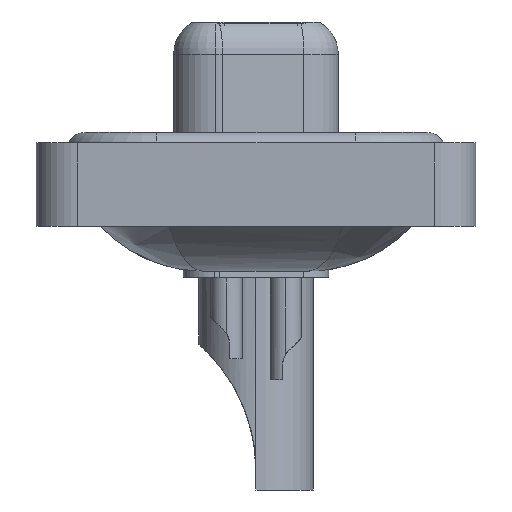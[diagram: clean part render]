
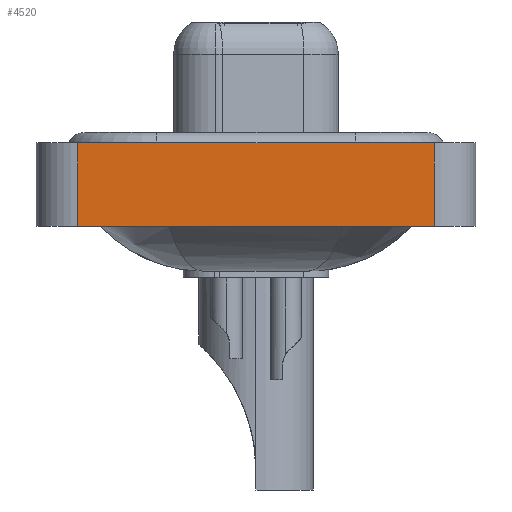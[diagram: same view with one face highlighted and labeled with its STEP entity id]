
A CAD part, left-side view. The second image highlights one B-rep face of the part: STEP entity #4520.
In plain terms, the highlighted planar face has unit normal (-1, 0, 0).
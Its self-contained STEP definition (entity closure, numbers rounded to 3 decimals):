
#196 = VERTEX_POINT ( 'NONE', #629 ) ;
#365 = DIRECTION ( 'NONE',  ( -1., 0., 0. ) ) ;
#629 = CARTESIAN_POINT ( 'NONE',  ( -7.3, -8.55, -3.6 ) ) ;
#1158 = CARTESIAN_POINT ( 'NONE',  ( -7.3, -8.55, -3.6 ) ) ;
#1205 = ORIENTED_EDGE ( 'NONE', *, *, #11827, .T. ) ;
#1836 = DIRECTION ( 'NONE',  ( 0., 0., 1. ) ) ;
#1920 = FACE_OUTER_BOUND ( 'NONE', #9299, .T. ) ;
#3502 = VECTOR ( 'NONE', #10788, 1000. ) ;
#3709 = ORIENTED_EDGE ( 'NONE', *, *, #17572, .F. ) ;
#4520 = ADVANCED_FACE ( 'NONE', ( #1920 ), #15809, .T. ) ;
#4964 = VECTOR ( 'NONE', #1836, 1000. ) ;
#5768 = VERTEX_POINT ( 'NONE', #18923 ) ;
#6378 = CARTESIAN_POINT ( 'NONE',  ( -7.3, -8.55, 0.4 ) ) ;
#6514 = CARTESIAN_POINT ( 'NONE',  ( -7.3, 8.55, 0.4 ) ) ;
#6992 = DIRECTION ( 'NONE',  ( 0., 0., 1. ) ) ;
#8396 = EDGE_CURVE ( 'NONE', #5768, #21709, #9965, .T. ) ;
#9299 = EDGE_LOOP ( 'NONE', ( #16265, #3709, #16435, #1205 ) ) ;
#9965 = LINE ( 'NONE', #22133, #19442 ) ;
#10788 = DIRECTION ( 'NONE',  ( 0., -1., 0. ) ) ;
#11827 = EDGE_CURVE ( 'NONE', #5768, #196, #20378, .T. ) ;
#12151 = CARTESIAN_POINT ( 'NONE',  ( -7.3, -8.55, -3.6 ) ) ;
#12922 = LINE ( 'NONE', #16337, #3502 ) ;
#13296 = DIRECTION ( 'NONE',  ( 0., -1., 0. ) ) ;
#13758 = LINE ( 'NONE', #17305, #4964 ) ;
#15809 = PLANE ( 'NONE',  #20923 ) ;
#16262 = VERTEX_POINT ( 'NONE', #6378 ) ;
#16265 = ORIENTED_EDGE ( 'NONE', *, *, #19578, .T. ) ;
#16337 = CARTESIAN_POINT ( 'NONE',  ( -7.3, -8.55, 0.4 ) ) ;
#16435 = ORIENTED_EDGE ( 'NONE', *, *, #8396, .F. ) ;
#17305 = CARTESIAN_POINT ( 'NONE',  ( -7.3, -8.55, -3.6 ) ) ;
#17572 = EDGE_CURVE ( 'NONE', #21709, #16262, #12922, .T. ) ;
#18539 = VECTOR ( 'NONE', #13296, 1000. ) ;
#18923 = CARTESIAN_POINT ( 'NONE',  ( -7.3, 8.55, -3.6 ) ) ;
#19442 = VECTOR ( 'NONE', #20309, 1000. ) ;
#19578 = EDGE_CURVE ( 'NONE', #196, #16262, #13758, .T. ) ;
#20309 = DIRECTION ( 'NONE',  ( 0., 0., 1. ) ) ;
#20378 = LINE ( 'NONE', #1158, #18539 ) ;
#20923 = AXIS2_PLACEMENT_3D ( 'NONE', #12151, #365, #6992 ) ;
#21709 = VERTEX_POINT ( 'NONE', #6514 ) ;
#22133 = CARTESIAN_POINT ( 'NONE',  ( -7.3, 8.55, -3.6 ) ) ;
